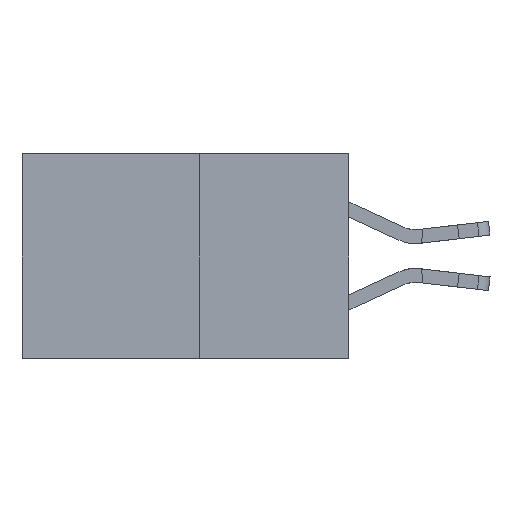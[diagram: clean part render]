
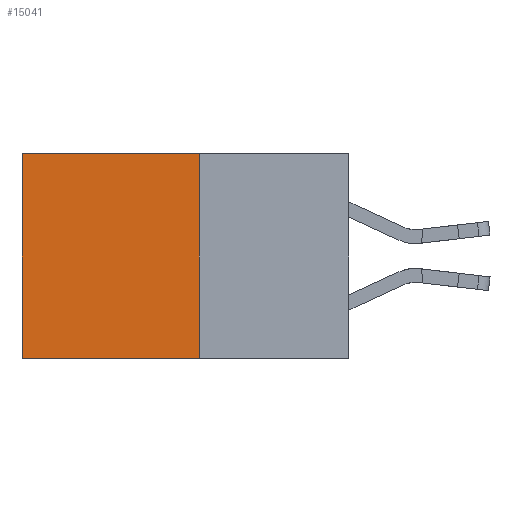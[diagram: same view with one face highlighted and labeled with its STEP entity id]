
A CAD part, left-side view. The second image highlights one B-rep face of the part: STEP entity #15041.
In plain terms, the highlighted planar face has unit normal (-1, 0, 0).
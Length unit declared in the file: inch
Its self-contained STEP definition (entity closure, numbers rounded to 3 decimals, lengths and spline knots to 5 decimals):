
#71 = ORIENTED_EDGE ( 'NONE', *, *, #19713, .F. ) ;
#137 = DIRECTION ( 'NONE',  ( 1., 0., 0. ) ) ;
#2346 = FACE_OUTER_BOUND ( 'NONE', #20173, .T. ) ;
#2348 = CARTESIAN_POINT ( 'NONE',  ( 0.277, 0.59, -0.37 ) ) ;
#2474 = VECTOR ( 'NONE', #4044, 39.37008 ) ;
#2706 = CARTESIAN_POINT ( 'NONE',  ( 0.277, 0.27, -0.37 ) ) ;
#2961 = LINE ( 'NONE', #20447, #11322 ) ;
#4044 = DIRECTION ( 'NONE',  ( 0., 0., -1. ) ) ;
#5087 = VERTEX_POINT ( 'NONE', #12713 ) ;
#5471 = DIRECTION ( 'NONE',  ( 0., 1., 0. ) ) ;
#6498 = ORIENTED_EDGE ( 'NONE', *, *, #6770, .F. ) ;
#6770 = EDGE_CURVE ( 'NONE', #13115, #19785, #8341, .T. ) ;
#7028 = CARTESIAN_POINT ( 'NONE',  ( 0.277, 0.27, -0.37 ) ) ;
#7720 = VECTOR ( 'NONE', #11631, 39.37008 ) ;
#8341 = LINE ( 'NONE', #2706, #12807 ) ;
#9003 = CARTESIAN_POINT ( 'NONE',  ( 0.277, 0.27, 0. ) ) ;
#9295 = LINE ( 'NONE', #19972, #7720 ) ;
#11296 = VERTEX_POINT ( 'NONE', #9003 ) ;
#11322 = VECTOR ( 'NONE', #5471, 39.37008 ) ;
#11631 = DIRECTION ( 'NONE',  ( 0., 0., -1. ) ) ;
#11790 = DIRECTION ( 'NONE',  ( 0., 0., -1. ) ) ;
#12333 = ORIENTED_EDGE ( 'NONE', *, *, #20004, .T. ) ;
#12713 = CARTESIAN_POINT ( 'NONE',  ( 0.277, 0.59, 0. ) ) ;
#12807 = VECTOR ( 'NONE', #19457, 39.37008 ) ;
#13115 = VERTEX_POINT ( 'NONE', #7028 ) ;
#14228 = ORIENTED_EDGE ( 'NONE', *, *, #18497, .T. ) ;
#15041 = ADVANCED_FACE ( 'NONE', ( #2346 ), #16728, .F. ) ;
#16728 = PLANE ( 'NONE',  #19104 ) ;
#18497 = EDGE_CURVE ( 'NONE', #11296, #5087, #2961, .T. ) ;
#19104 = AXIS2_PLACEMENT_3D ( 'NONE', #20119, #137, #11790 ) ;
#19457 = DIRECTION ( 'NONE',  ( 0., 1., 0. ) ) ;
#19713 = EDGE_CURVE ( 'NONE', #11296, #13115, #9295, .T. ) ;
#19785 = VERTEX_POINT ( 'NONE', #20187 ) ;
#19972 = CARTESIAN_POINT ( 'NONE',  ( 0.277, 0.27, -0.37 ) ) ;
#20004 = EDGE_CURVE ( 'NONE', #5087, #19785, #20267, .T. ) ;
#20119 = CARTESIAN_POINT ( 'NONE',  ( 0.277, 0.27, -0.37 ) ) ;
#20173 = EDGE_LOOP ( 'NONE', ( #12333, #6498, #71, #14228 ) ) ;
#20187 = CARTESIAN_POINT ( 'NONE',  ( 0.277, 0.59, -0.37 ) ) ;
#20267 = LINE ( 'NONE', #2348, #2474 ) ;
#20447 = CARTESIAN_POINT ( 'NONE',  ( 0.277, 0.27, 0. ) ) ;
